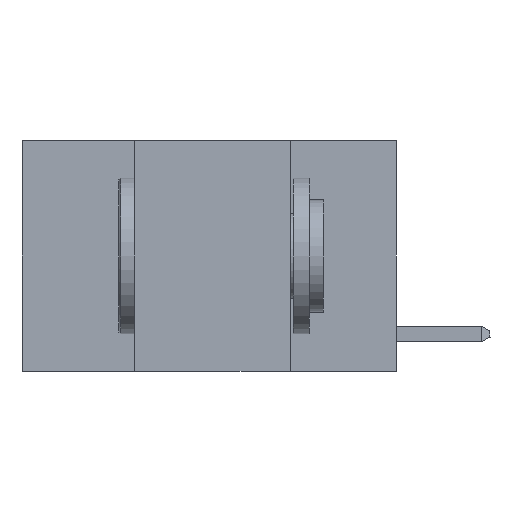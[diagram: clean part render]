
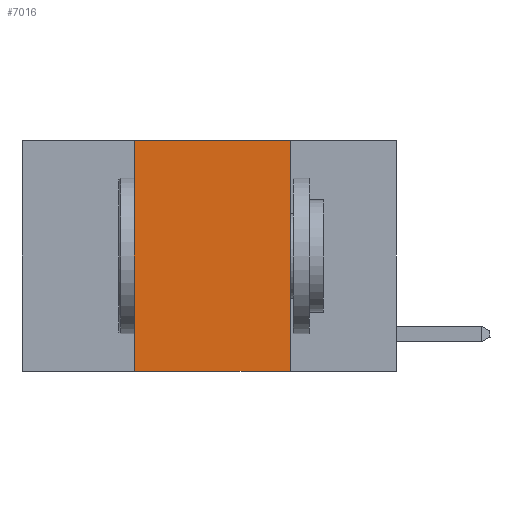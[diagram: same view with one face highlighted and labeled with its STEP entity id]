
A CAD part, left-side view. The second image highlights one B-rep face of the part: STEP entity #7016.
In plain terms, the highlighted planar face has unit normal (-1, 0, 0).
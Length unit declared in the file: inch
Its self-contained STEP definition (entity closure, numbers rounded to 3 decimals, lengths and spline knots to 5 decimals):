
#158 = CARTESIAN_POINT ( 'NONE',  ( 0., 0.42, -0.37 ) ) ;
#283 = CARTESIAN_POINT ( 'NONE',  ( 0., 0.6, 0. ) ) ;
#419 = DIRECTION ( 'NONE',  ( 0., -1., 0. ) ) ;
#808 = CARTESIAN_POINT ( 'NONE',  ( 0., 0.6, 0. ) ) ;
#1859 = LINE ( 'NONE', #7881, #9242 ) ;
#2293 = EDGE_CURVE ( 'NONE', #4427, #7471, #6800, .T. ) ;
#2341 = LINE ( 'NONE', #3717, #8780 ) ;
#2353 = VECTOR ( 'NONE', #4450, 39.37008 ) ;
#2508 = VECTOR ( 'NONE', #419, 39.37008 ) ;
#2585 = DIRECTION ( 'NONE',  ( 0., 0., -1. ) ) ;
#3413 = CARTESIAN_POINT ( 'NONE',  ( 0., 0.17, 0. ) ) ;
#3455 = DIRECTION ( 'NONE',  ( 0., 0., 1. ) ) ;
#3717 = CARTESIAN_POINT ( 'NONE',  ( 0., 0.17, 0. ) ) ;
#4041 = AXIS2_PLACEMENT_3D ( 'NONE', #283, #6352, #2585 ) ;
#4427 = VERTEX_POINT ( 'NONE', #8414 ) ;
#4450 = DIRECTION ( 'NONE',  ( 0., -1., 0. ) ) ;
#4938 = ORIENTED_EDGE ( 'NONE', *, *, #5440, .T. ) ;
#5036 = EDGE_CURVE ( 'NONE', #7471, #7645, #2341, .T. ) ;
#5197 = CARTESIAN_POINT ( 'NONE',  ( 0., 0.6, -0.37 ) ) ;
#5440 = EDGE_CURVE ( 'NONE', #5843, #7645, #6613, .T. ) ;
#5843 = VERTEX_POINT ( 'NONE', #158 ) ;
#6352 = DIRECTION ( 'NONE',  ( 1., 0., 0. ) ) ;
#6613 = LINE ( 'NONE', #5197, #2508 ) ;
#6654 = EDGE_CURVE ( 'NONE', #5843, #4427, #1859, .T. ) ;
#6731 = ORIENTED_EDGE ( 'NONE', *, *, #5036, .F. ) ;
#6800 = LINE ( 'NONE', #808, #2353 ) ;
#7016 = ADVANCED_FACE ( 'NONE', ( #7123 ), #7070, .F. ) ;
#7070 = PLANE ( 'NONE',  #4041 ) ;
#7123 = FACE_OUTER_BOUND ( 'NONE', #9449, .T. ) ;
#7385 = ORIENTED_EDGE ( 'NONE', *, *, #6654, .F. ) ;
#7471 = VERTEX_POINT ( 'NONE', #3413 ) ;
#7645 = VERTEX_POINT ( 'NONE', #9281 ) ;
#7881 = CARTESIAN_POINT ( 'NONE',  ( 0., 0.42, 0. ) ) ;
#8272 = DIRECTION ( 'NONE',  ( 0., 0., -1. ) ) ;
#8414 = CARTESIAN_POINT ( 'NONE',  ( 0., 0.42, 0. ) ) ;
#8780 = VECTOR ( 'NONE', #8272, 39.37008 ) ;
#9242 = VECTOR ( 'NONE', #3455, 39.37008 ) ;
#9281 = CARTESIAN_POINT ( 'NONE',  ( 0., 0.17, -0.37 ) ) ;
#9339 = ORIENTED_EDGE ( 'NONE', *, *, #2293, .F. ) ;
#9449 = EDGE_LOOP ( 'NONE', ( #6731, #9339, #7385, #4938 ) ) ;
